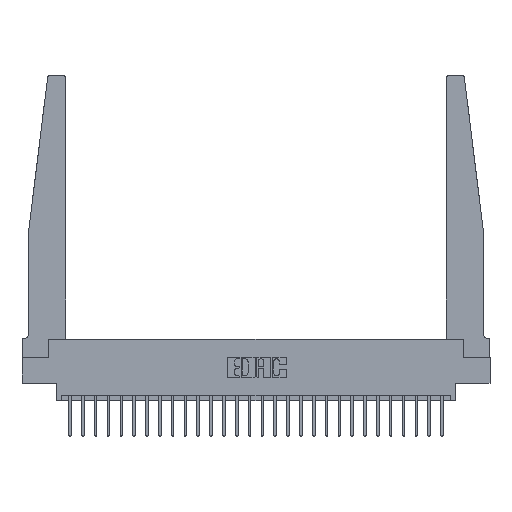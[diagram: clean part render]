
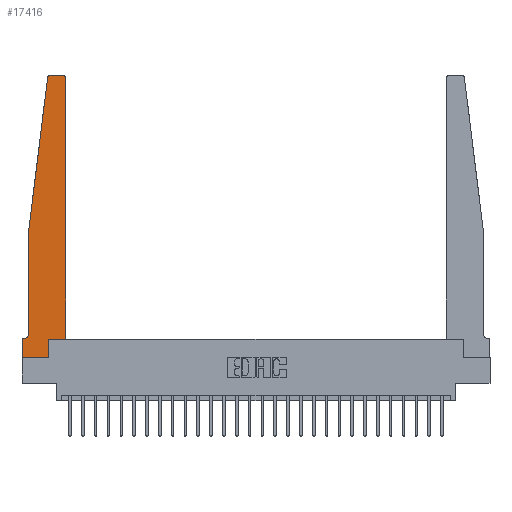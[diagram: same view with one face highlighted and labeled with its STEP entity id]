
A CAD part, top view. The second image highlights one B-rep face of the part: STEP entity #17416.
In plain terms, the highlighted planar face has unit normal (0, 0, 1).
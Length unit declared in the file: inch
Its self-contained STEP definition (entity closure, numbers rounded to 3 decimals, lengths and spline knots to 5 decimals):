
#129 = CARTESIAN_POINT ( 'NONE',  ( 0.395, 2.72, 0.37 ) ) ;
#234 = LINE ( 'NONE', #357, #13161 ) ;
#355 = CARTESIAN_POINT ( 'NONE',  ( 0.015, 0.1875, 0.37 ) ) ;
#357 = CARTESIAN_POINT ( 'NONE',  ( 0.25, 2.75, 0.37 ) ) ;
#443 = LINE ( 'NONE', #1422, #16590 ) ;
#1422 = CARTESIAN_POINT ( 'NONE',  ( 0.425, 0.18, 0.37 ) ) ;
#1479 = LINE ( 'NONE', #24375, #6830 ) ;
#1486 = EDGE_CURVE ( 'NONE', #15548, #16666, #3700, .T. ) ;
#1912 = VECTOR ( 'NONE', #5400, 39.37008 ) ;
#2175 = DIRECTION ( 'NONE',  ( 1., 0., 0. ) ) ;
#2234 = AXIS2_PLACEMENT_3D ( 'NONE', #3660, #17810, #5695 ) ;
#2437 = DIRECTION ( 'NONE',  ( 1., 0., 0. ) ) ;
#2727 = ORIENTED_EDGE ( 'NONE', *, *, #10404, .T. ) ;
#2802 = CIRCLE ( 'NONE', #25667, 0.03 ) ;
#2892 = CARTESIAN_POINT ( 'NONE',  ( 0.065, 1.25, 0.37 ) ) ;
#3061 = EDGE_CURVE ( 'NONE', #16921, #25617, #443, .T. ) ;
#3660 = CARTESIAN_POINT ( 'NONE',  ( 0.27653, 2.72, 0.37 ) ) ;
#3700 = LINE ( 'NONE', #19413, #24545 ) ;
#4299 = ORIENTED_EDGE ( 'NONE', *, *, #16314, .T. ) ;
#5012 = CARTESIAN_POINT ( 'NONE',  ( 0.425, 0.18, 0.37 ) ) ;
#5144 = CARTESIAN_POINT ( 'NONE',  ( 0.24675, 2.72367, 0.37 ) ) ;
#5400 = DIRECTION ( 'NONE',  ( -0.122, -0.992, 0. ) ) ;
#5571 = ORIENTED_EDGE ( 'NONE', *, *, #24211, .T. ) ;
#5695 = DIRECTION ( 'NONE',  ( 1., 0., 0. ) ) ;
#5977 = CARTESIAN_POINT ( 'NONE',  ( 0.2605, 0.18, 0.37 ) ) ;
#6656 = LINE ( 'NONE', #17521, #1912 ) ;
#6830 = VECTOR ( 'NONE', #18223, 39.37008 ) ;
#6981 = EDGE_CURVE ( 'NONE', #23632, #12001, #234, .T. ) ;
#7260 = DIRECTION ( 'NONE',  ( 0., -1., 0. ) ) ;
#8484 = FACE_OUTER_BOUND ( 'NONE', #13609, .T. ) ;
#9521 = CARTESIAN_POINT ( 'NONE',  ( 0.015, 0.2375, 0.37 ) ) ;
#10404 = EDGE_CURVE ( 'NONE', #25617, #25320, #24610, .T. ) ;
#10416 = AXIS2_PLACEMENT_3D ( 'NONE', #9521, #23703, #11564 ) ;
#10417 = CARTESIAN_POINT ( 'NONE',  ( 0., 0., 0.37 ) ) ;
#10617 = DIRECTION ( 'NONE',  ( 0., 0., 1. ) ) ;
#10709 = EDGE_CURVE ( 'NONE', #25320, #23632, #2802, .T. ) ;
#10822 = CARTESIAN_POINT ( 'NONE',  ( 0.2605, 0.18, 0.37 ) ) ;
#11564 = DIRECTION ( 'NONE',  ( -1., 0., 0. ) ) ;
#11737 = CARTESIAN_POINT ( 'NONE',  ( 0., 0., 0.37 ) ) ;
#12001 = VERTEX_POINT ( 'NONE', #15866 ) ;
#12172 = ORIENTED_EDGE ( 'NONE', *, *, #15984, .T. ) ;
#12214 = VECTOR ( 'NONE', #18534, 39.37008 ) ;
#12388 = CARTESIAN_POINT ( 'NONE',  ( 0.065, 0.1875, 0.37 ) ) ;
#13161 = VECTOR ( 'NONE', #16544, 39.37008 ) ;
#13516 = DIRECTION ( 'NONE',  ( 1., 0., 0. ) ) ;
#13609 = EDGE_LOOP ( 'NONE', ( #19181, #4299, #24846, #15048, #16334, #5571, #17609, #12172, #23583, #22952, #2727, #17314 ) ) ;
#13936 = EDGE_CURVE ( 'NONE', #21132, #16921, #22559, .T. ) ;
#14146 = CARTESIAN_POINT ( 'NONE',  ( 0.425, 2.72, 0.37 ) ) ;
#14277 = DIRECTION ( 'NONE',  ( 0., 0., 1. ) ) ;
#14379 = CARTESIAN_POINT ( 'NONE',  ( 0.2605, 0., 0.37 ) ) ;
#15048 = ORIENTED_EDGE ( 'NONE', *, *, #1486, .T. ) ;
#15539 = VECTOR ( 'NONE', #2437, 39.37008 ) ;
#15548 = VERTEX_POINT ( 'NONE', #2892 ) ;
#15866 = CARTESIAN_POINT ( 'NONE',  ( 0.27653, 2.75, 0.37 ) ) ;
#15984 = EDGE_CURVE ( 'NONE', #24670, #21132, #20923, .T. ) ;
#16144 = DIRECTION ( 'NONE',  ( 0., 1., 0. ) ) ;
#16314 = EDGE_CURVE ( 'NONE', #12001, #20017, #18699, .T. ) ;
#16334 = ORIENTED_EDGE ( 'NONE', *, *, #24598, .T. ) ;
#16544 = DIRECTION ( 'NONE',  ( -1., 0., 0. ) ) ;
#16590 = VECTOR ( 'NONE', #13516, 39.37008 ) ;
#16666 = VERTEX_POINT ( 'NONE', #19119 ) ;
#16921 = VERTEX_POINT ( 'NONE', #10822 ) ;
#16996 = AXIS2_PLACEMENT_3D ( 'NONE', #22770, #10617, #24786 ) ;
#17019 = EDGE_CURVE ( 'NONE', #20017, #15548, #6656, .T. ) ;
#17206 = VECTOR ( 'NONE', #16144, 39.37008 ) ;
#17314 = ORIENTED_EDGE ( 'NONE', *, *, #10709, .T. ) ;
#17416 = ADVANCED_FACE ( 'NONE', ( #8484 ), #24699, .T. ) ;
#17521 = CARTESIAN_POINT ( 'NONE',  ( 0.065, 1.25, 0.37 ) ) ;
#17609 = ORIENTED_EDGE ( 'NONE', *, *, #20392, .T. ) ;
#17810 = DIRECTION ( 'NONE',  ( 0., 0., 1. ) ) ;
#18223 = DIRECTION ( 'NONE',  ( 0., -1., 0. ) ) ;
#18534 = DIRECTION ( 'NONE',  ( -1., 0., 0. ) ) ;
#18585 = VERTEX_POINT ( 'NONE', #355 ) ;
#18699 = CIRCLE ( 'NONE', #2234, 0.03 ) ;
#18808 = VERTEX_POINT ( 'NONE', #25159 ) ;
#19119 = CARTESIAN_POINT ( 'NONE',  ( 0.065, 0.2375, 0.37 ) ) ;
#19181 = ORIENTED_EDGE ( 'NONE', *, *, #6981, .T. ) ;
#19279 = VECTOR ( 'NONE', #23198, 39.37008 ) ;
#19413 = CARTESIAN_POINT ( 'NONE',  ( 0.065, 1.25, 0.37 ) ) ;
#20017 = VERTEX_POINT ( 'NONE', #5144 ) ;
#20142 = CIRCLE ( 'NONE', #10416, 0.05 ) ;
#20392 = EDGE_CURVE ( 'NONE', #18808, #24670, #1479, .T. ) ;
#20923 = LINE ( 'NONE', #10417, #15539 ) ;
#21132 = VERTEX_POINT ( 'NONE', #14379 ) ;
#21307 = CARTESIAN_POINT ( 'NONE',  ( 0.425, 0.18, 0.37 ) ) ;
#22559 = LINE ( 'NONE', #5977, #17206 ) ;
#22770 = CARTESIAN_POINT ( 'NONE',  ( 0., 0.1875, 0.37 ) ) ;
#22952 = ORIENTED_EDGE ( 'NONE', *, *, #3061, .T. ) ;
#22997 = LINE ( 'NONE', #12388, #12214 ) ;
#23198 = DIRECTION ( 'NONE',  ( 0., 1., 0. ) ) ;
#23583 = ORIENTED_EDGE ( 'NONE', *, *, #13936, .T. ) ;
#23632 = VERTEX_POINT ( 'NONE', #24975 ) ;
#23703 = DIRECTION ( 'NONE',  ( 0., 0., -1. ) ) ;
#24211 = EDGE_CURVE ( 'NONE', #18585, #18808, #22997, .T. ) ;
#24375 = CARTESIAN_POINT ( 'NONE',  ( 0., 0., 0.37 ) ) ;
#24545 = VECTOR ( 'NONE', #7260, 39.37008 ) ;
#24598 = EDGE_CURVE ( 'NONE', #16666, #18585, #20142, .T. ) ;
#24610 = LINE ( 'NONE', #5012, #19279 ) ;
#24670 = VERTEX_POINT ( 'NONE', #11737 ) ;
#24699 = PLANE ( 'NONE',  #16996 ) ;
#24786 = DIRECTION ( 'NONE',  ( 1., 0., 0. ) ) ;
#24846 = ORIENTED_EDGE ( 'NONE', *, *, #17019, .T. ) ;
#24975 = CARTESIAN_POINT ( 'NONE',  ( 0.395, 2.75, 0.37 ) ) ;
#25159 = CARTESIAN_POINT ( 'NONE',  ( 0., 0.1875, 0.37 ) ) ;
#25320 = VERTEX_POINT ( 'NONE', #14146 ) ;
#25617 = VERTEX_POINT ( 'NONE', #21307 ) ;
#25667 = AXIS2_PLACEMENT_3D ( 'NONE', #129, #14277, #2175 ) ;
